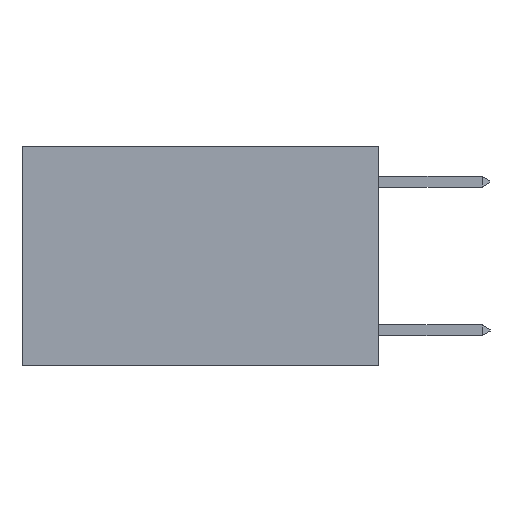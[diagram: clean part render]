
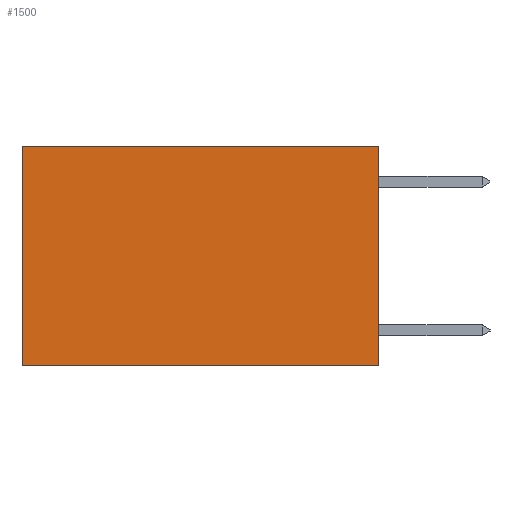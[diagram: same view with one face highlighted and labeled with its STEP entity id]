
A CAD part, left-side view. The second image highlights one B-rep face of the part: STEP entity #1500.
In plain terms, the highlighted planar face has unit normal (-1, 0, 0).
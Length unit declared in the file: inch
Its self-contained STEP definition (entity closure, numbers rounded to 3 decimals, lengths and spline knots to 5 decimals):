
#500 = VECTOR ( 'NONE', #3235, 39.37008 ) ;
#789 = DIRECTION ( 'NONE',  ( 0., 1., 0. ) ) ;
#805 = VERTEX_POINT ( 'NONE', #7787 ) ;
#1095 = CARTESIAN_POINT ( 'NONE',  ( 0.2625, 0.6, -0.37 ) ) ;
#1472 = CARTESIAN_POINT ( 'NONE',  ( 0.2625, 0., -0.37 ) ) ;
#1500 = ADVANCED_FACE ( 'NONE', ( #4142 ), #8199, .F. ) ;
#1516 = VERTEX_POINT ( 'NONE', #2477 ) ;
#1769 = DIRECTION ( 'NONE',  ( 0., 0., -1. ) ) ;
#1831 = CARTESIAN_POINT ( 'NONE',  ( 0.2625, 0., 0. ) ) ;
#2097 = CARTESIAN_POINT ( 'NONE',  ( 0.2625, 0., 0. ) ) ;
#2254 = DIRECTION ( 'NONE',  ( 0., 0., -1. ) ) ;
#2477 = CARTESIAN_POINT ( 'NONE',  ( 0.2625, 0.6, 0. ) ) ;
#2579 = CARTESIAN_POINT ( 'NONE',  ( 0.2625, 0.6, 0. ) ) ;
#2622 = DIRECTION ( 'NONE',  ( 1., 0., 0. ) ) ;
#3235 = DIRECTION ( 'NONE',  ( 0., 0., -1. ) ) ;
#3364 = CARTESIAN_POINT ( 'NONE',  ( 0.2625, 0., 0. ) ) ;
#3683 = EDGE_LOOP ( 'NONE', ( #4384, #5377, #5290, #7898 ) ) ;
#4142 = FACE_OUTER_BOUND ( 'NONE', #3683, .T. ) ;
#4311 = VECTOR ( 'NONE', #6895, 39.37008 ) ;
#4345 = EDGE_CURVE ( 'NONE', #8373, #1516, #6017, .T. ) ;
#4384 = ORIENTED_EDGE ( 'NONE', *, *, #8377, .T. ) ;
#5290 = ORIENTED_EDGE ( 'NONE', *, *, #5568, .F. ) ;
#5377 = ORIENTED_EDGE ( 'NONE', *, *, #7357, .F. ) ;
#5528 = LINE ( 'NONE', #2579, #500 ) ;
#5568 = EDGE_CURVE ( 'NONE', #8373, #805, #8107, .T. ) ;
#6017 = LINE ( 'NONE', #3364, #4311 ) ;
#6445 = CARTESIAN_POINT ( 'NONE',  ( 0.2625, 0., 0. ) ) ;
#6468 = VERTEX_POINT ( 'NONE', #1095 ) ;
#6566 = LINE ( 'NONE', #1472, #8077 ) ;
#6895 = DIRECTION ( 'NONE',  ( 0., 1., 0. ) ) ;
#7357 = EDGE_CURVE ( 'NONE', #805, #6468, #6566, .T. ) ;
#7787 = CARTESIAN_POINT ( 'NONE',  ( 0.2625, 0., -0.37 ) ) ;
#7893 = VECTOR ( 'NONE', #2254, 39.37008 ) ;
#7898 = ORIENTED_EDGE ( 'NONE', *, *, #4345, .T. ) ;
#7968 = AXIS2_PLACEMENT_3D ( 'NONE', #1831, #2622, #1769 ) ;
#8077 = VECTOR ( 'NONE', #789, 39.37008 ) ;
#8107 = LINE ( 'NONE', #2097, #7893 ) ;
#8199 = PLANE ( 'NONE',  #7968 ) ;
#8373 = VERTEX_POINT ( 'NONE', #6445 ) ;
#8377 = EDGE_CURVE ( 'NONE', #1516, #6468, #5528, .T. ) ;
